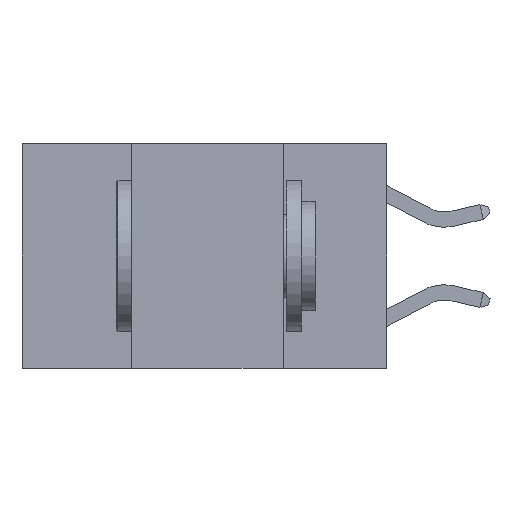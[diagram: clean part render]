
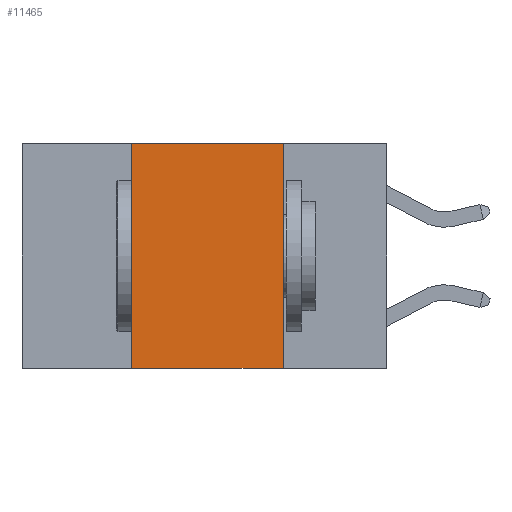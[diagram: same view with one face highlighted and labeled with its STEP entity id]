
A CAD part, left-side view. The second image highlights one B-rep face of the part: STEP entity #11465.
In plain terms, the highlighted planar face has unit normal (-1, 0, 0).
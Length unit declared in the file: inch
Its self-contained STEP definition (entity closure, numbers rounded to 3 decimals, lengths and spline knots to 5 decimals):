
#119 = CARTESIAN_POINT ( 'NONE',  ( 0., 0.42, 0. ) ) ;
#587 = VECTOR ( 'NONE', #15700, 39.37008 ) ;
#603 = VERTEX_POINT ( 'NONE', #4033 ) ;
#1903 = LINE ( 'NONE', #14804, #6683 ) ;
#2490 = ORIENTED_EDGE ( 'NONE', *, *, #5953, .F. ) ;
#3415 = CARTESIAN_POINT ( 'NONE',  ( 0., 0.42, -0.37 ) ) ;
#3914 = DIRECTION ( 'NONE',  ( 0., 0., 1. ) ) ;
#4033 = CARTESIAN_POINT ( 'NONE',  ( 0., 0.17, -0.37 ) ) ;
#4355 = PLANE ( 'NONE',  #13927 ) ;
#4412 = VERTEX_POINT ( 'NONE', #119 ) ;
#5333 = LINE ( 'NONE', #6625, #587 ) ;
#5953 = EDGE_CURVE ( 'NONE', #4412, #7157, #18718, .T. ) ;
#6625 = CARTESIAN_POINT ( 'NONE',  ( 0., 0.6, -0.37 ) ) ;
#6683 = VECTOR ( 'NONE', #3914, 39.37008 ) ;
#7157 = VERTEX_POINT ( 'NONE', #9158 ) ;
#7202 = VECTOR ( 'NONE', #12750, 39.37008 ) ;
#7204 = CARTESIAN_POINT ( 'NONE',  ( 0., 0.17, 0. ) ) ;
#7281 = ORIENTED_EDGE ( 'NONE', *, *, #7570, .F. ) ;
#7570 = EDGE_CURVE ( 'NONE', #8324, #4412, #1903, .T. ) ;
#8001 = DIRECTION ( 'NONE',  ( 0., 0., -1. ) ) ;
#8324 = VERTEX_POINT ( 'NONE', #3415 ) ;
#9158 = CARTESIAN_POINT ( 'NONE',  ( 0., 0.17, 0. ) ) ;
#10877 = DIRECTION ( 'NONE',  ( 0., -1., 0. ) ) ;
#11465 = ADVANCED_FACE ( 'NONE', ( #18734 ), #4355, .F. ) ;
#12750 = DIRECTION ( 'NONE',  ( 0., 0., -1. ) ) ;
#12755 = ORIENTED_EDGE ( 'NONE', *, *, #14532, .T. ) ;
#13053 = EDGE_LOOP ( 'NONE', ( #16366, #2490, #7281, #12755 ) ) ;
#13927 = AXIS2_PLACEMENT_3D ( 'NONE', #15237, #18864, #8001 ) ;
#14532 = EDGE_CURVE ( 'NONE', #8324, #603, #5333, .T. ) ;
#14804 = CARTESIAN_POINT ( 'NONE',  ( 0., 0.42, 0. ) ) ;
#15237 = CARTESIAN_POINT ( 'NONE',  ( 0., 0.6, 0. ) ) ;
#15700 = DIRECTION ( 'NONE',  ( 0., -1., 0. ) ) ;
#16366 = ORIENTED_EDGE ( 'NONE', *, *, #21414, .F. ) ;
#17412 = LINE ( 'NONE', #7204, #7202 ) ;
#18718 = LINE ( 'NONE', #19908, #22829 ) ;
#18734 = FACE_OUTER_BOUND ( 'NONE', #13053, .T. ) ;
#18864 = DIRECTION ( 'NONE',  ( 1., 0., 0. ) ) ;
#19908 = CARTESIAN_POINT ( 'NONE',  ( 0., 0.6, 0. ) ) ;
#21414 = EDGE_CURVE ( 'NONE', #7157, #603, #17412, .T. ) ;
#22829 = VECTOR ( 'NONE', #10877, 39.37008 ) ;
